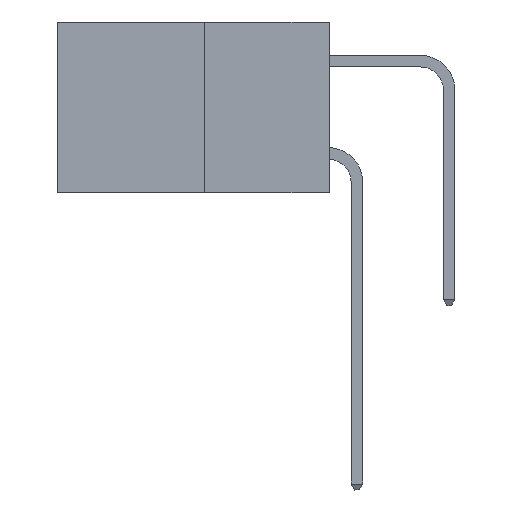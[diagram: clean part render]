
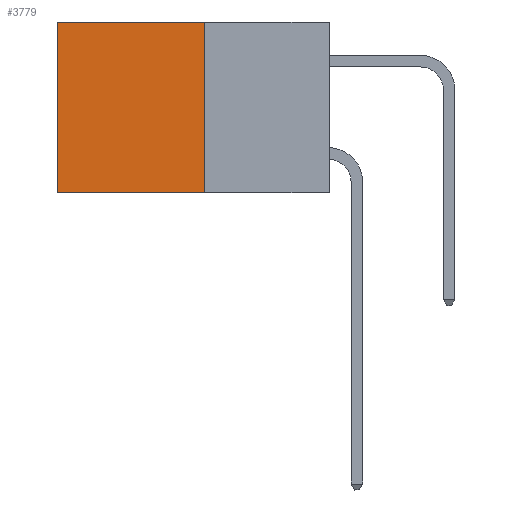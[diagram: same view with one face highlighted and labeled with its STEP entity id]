
A CAD part, left-side view. The second image highlights one B-rep face of the part: STEP entity #3779.
In plain terms, the highlighted planar face has unit normal (-1, 0, 0).
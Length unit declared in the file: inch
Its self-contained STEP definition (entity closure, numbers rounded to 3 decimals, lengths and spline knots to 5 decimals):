
#223 = EDGE_LOOP ( 'NONE', ( #13535, #15318, #320, #14736 ) ) ;
#320 = ORIENTED_EDGE ( 'NONE', *, *, #19576, .F. ) ;
#957 = CARTESIAN_POINT ( 'NONE',  ( 0.277, 0.27, -0.37 ) ) ;
#968 = VERTEX_POINT ( 'NONE', #5012 ) ;
#1774 = VECTOR ( 'NONE', #10616, 39.37008 ) ;
#2005 = LINE ( 'NONE', #22284, #6514 ) ;
#2580 = LINE ( 'NONE', #20380, #12223 ) ;
#2911 = DIRECTION ( 'NONE',  ( 0., 1., 0. ) ) ;
#3779 = ADVANCED_FACE ( 'NONE', ( #22481 ), #22895, .F. ) ;
#5012 = CARTESIAN_POINT ( 'NONE',  ( 0.277, 0.27, 0. ) ) ;
#5726 = CARTESIAN_POINT ( 'NONE',  ( 0.277, 0.59, -0.37 ) ) ;
#5775 = VERTEX_POINT ( 'NONE', #5726 ) ;
#6514 = VECTOR ( 'NONE', #12917, 39.37008 ) ;
#8162 = VECTOR ( 'NONE', #2911, 39.37008 ) ;
#8667 = AXIS2_PLACEMENT_3D ( 'NONE', #19570, #18359, #20220 ) ;
#8690 = CARTESIAN_POINT ( 'NONE',  ( 0.277, 0.27, 0. ) ) ;
#10616 = DIRECTION ( 'NONE',  ( 0., 1., 0. ) ) ;
#11206 = VERTEX_POINT ( 'NONE', #17272 ) ;
#12223 = VECTOR ( 'NONE', #24060, 39.37008 ) ;
#12917 = DIRECTION ( 'NONE',  ( 0., 0., -1. ) ) ;
#13535 = ORIENTED_EDGE ( 'NONE', *, *, #19541, .T. ) ;
#14736 = ORIENTED_EDGE ( 'NONE', *, *, #15277, .T. ) ;
#15217 = CARTESIAN_POINT ( 'NONE',  ( 0.277, 0.27, -0.37 ) ) ;
#15277 = EDGE_CURVE ( 'NONE', #968, #11206, #17054, .T. ) ;
#15318 = ORIENTED_EDGE ( 'NONE', *, *, #22562, .F. ) ;
#17054 = LINE ( 'NONE', #8690, #1774 ) ;
#17272 = CARTESIAN_POINT ( 'NONE',  ( 0.277, 0.59, 0. ) ) ;
#17725 = LINE ( 'NONE', #957, #8162 ) ;
#18359 = DIRECTION ( 'NONE',  ( 1., 0., 0. ) ) ;
#19541 = EDGE_CURVE ( 'NONE', #11206, #5775, #2580, .T. ) ;
#19570 = CARTESIAN_POINT ( 'NONE',  ( 0.277, 0.27, -0.37 ) ) ;
#19576 = EDGE_CURVE ( 'NONE', #968, #21602, #2005, .T. ) ;
#20220 = DIRECTION ( 'NONE',  ( 0., 0., -1. ) ) ;
#20380 = CARTESIAN_POINT ( 'NONE',  ( 0.277, 0.59, -0.37 ) ) ;
#21602 = VERTEX_POINT ( 'NONE', #15217 ) ;
#22284 = CARTESIAN_POINT ( 'NONE',  ( 0.277, 0.27, -0.37 ) ) ;
#22481 = FACE_OUTER_BOUND ( 'NONE', #223, .T. ) ;
#22562 = EDGE_CURVE ( 'NONE', #21602, #5775, #17725, .T. ) ;
#22895 = PLANE ( 'NONE',  #8667 ) ;
#24060 = DIRECTION ( 'NONE',  ( 0., 0., -1. ) ) ;
